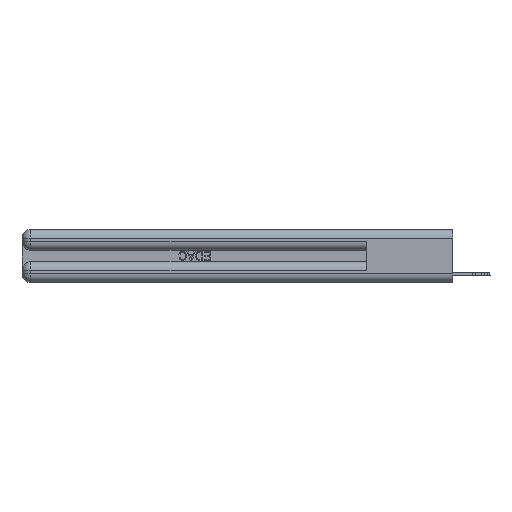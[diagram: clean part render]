
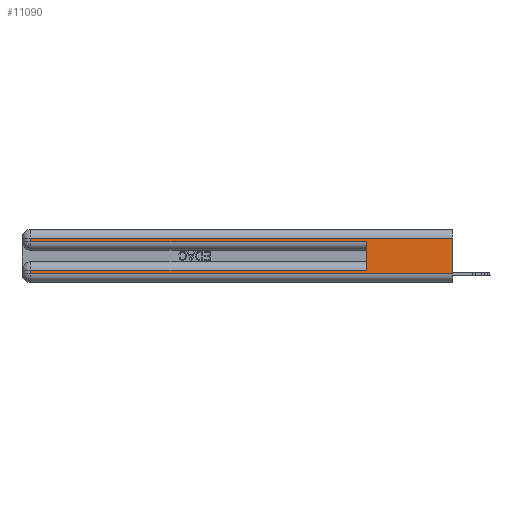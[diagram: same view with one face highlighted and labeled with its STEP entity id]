
A CAD part, left-side view. The second image highlights one B-rep face of the part: STEP entity #11090.
In plain terms, the highlighted planar face has unit normal (-1, 0, 0).
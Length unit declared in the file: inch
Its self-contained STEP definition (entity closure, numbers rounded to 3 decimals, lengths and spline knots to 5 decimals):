
#263 = CARTESIAN_POINT ( 'NONE',  ( 0., 0., 0.285 ) ) ;
#1308 = ORIENTED_EDGE ( 'NONE', *, *, #21689, .T. ) ;
#2280 = DIRECTION ( 'NONE',  ( 0., 1., 0. ) ) ;
#2573 = ORIENTED_EDGE ( 'NONE', *, *, #19271, .F. ) ;
#2733 = VECTOR ( 'NONE', #10560, 39.37008 ) ;
#3827 = CARTESIAN_POINT ( 'NONE',  ( 0., 2.94, 0.37 ) ) ;
#4783 = ORIENTED_EDGE ( 'NONE', *, *, #11124, .T. ) ;
#4931 = DIRECTION ( 'NONE',  ( 0., 0., -1. ) ) ;
#5399 = CARTESIAN_POINT ( 'NONE',  ( 0., 0., 0.06 ) ) ;
#5500 = VERTEX_POINT ( 'NONE', #27693 ) ;
#5963 = VECTOR ( 'NONE', #8279, 39.37008 ) ;
#7023 = CARTESIAN_POINT ( 'NONE',  ( 0., 0., 0.37 ) ) ;
#7099 = CARTESIAN_POINT ( 'NONE',  ( 0., 2.94, 0.37 ) ) ;
#8279 = DIRECTION ( 'NONE',  ( 0., 0., 1. ) ) ;
#8488 = VECTOR ( 'NONE', #12226, 39.37008 ) ;
#8755 = LINE ( 'NONE', #18513, #5963 ) ;
#8760 = VECTOR ( 'NONE', #2280, 39.37008 ) ;
#10560 = DIRECTION ( 'NONE',  ( 0., 1., 0. ) ) ;
#11020 = VERTEX_POINT ( 'NONE', #23036 ) ;
#11090 = ADVANCED_FACE ( 'NONE', ( #18244 ), #15538, .F. ) ;
#11124 = EDGE_CURVE ( 'NONE', #5500, #11020, #12974, .T. ) ;
#12226 = DIRECTION ( 'NONE',  ( 0., 0., -1. ) ) ;
#12974 = LINE ( 'NONE', #22556, #2733 ) ;
#13335 = ORIENTED_EDGE ( 'NONE', *, *, #22567, .T. ) ;
#13563 = EDGE_CURVE ( 'NONE', #30254, #25955, #14953, .T. ) ;
#14432 = CARTESIAN_POINT ( 'NONE',  ( 0., 2.94, 0.285 ) ) ;
#14953 = LINE ( 'NONE', #7099, #8488 ) ;
#15154 = VERTEX_POINT ( 'NONE', #22585 ) ;
#15222 = EDGE_CURVE ( 'NONE', #25955, #22639, #30396, .T. ) ;
#15402 = ORIENTED_EDGE ( 'NONE', *, *, #15222, .T. ) ;
#15538 = PLANE ( 'NONE',  #28278 ) ;
#16202 = EDGE_CURVE ( 'NONE', #15154, #21276, #8755, .T. ) ;
#17010 = EDGE_CURVE ( 'NONE', #11020, #22063, #25745, .T. ) ;
#17110 = DIRECTION ( 'NONE',  ( 0., -1., 0. ) ) ;
#18120 = EDGE_LOOP ( 'NONE', ( #2573, #4783, #28640, #13335, #25942, #1308, #27802, #15402 ) ) ;
#18244 = FACE_OUTER_BOUND ( 'NONE', #18120, .T. ) ;
#18513 = CARTESIAN_POINT ( 'NONE',  ( 0., 0.6, 0.145 ) ) ;
#18586 = CARTESIAN_POINT ( 'NONE',  ( 0., 0., 0.06 ) ) ;
#19181 = LINE ( 'NONE', #7023, #30069 ) ;
#19271 = EDGE_CURVE ( 'NONE', #5500, #22639, #19181, .T. ) ;
#19563 = LINE ( 'NONE', #24206, #8760 ) ;
#19778 = VECTOR ( 'NONE', #28012, 39.37008 ) ;
#21276 = VERTEX_POINT ( 'NONE', #24384 ) ;
#21689 = EDGE_CURVE ( 'NONE', #15154, #30254, #19563, .T. ) ;
#21897 = CARTESIAN_POINT ( 'NONE',  ( 0., 2.94, 0.085 ) ) ;
#22063 = VERTEX_POINT ( 'NONE', #14432 ) ;
#22556 = CARTESIAN_POINT ( 'NONE',  ( 0., 0., 0.31 ) ) ;
#22567 = EDGE_CURVE ( 'NONE', #22063, #21276, #24614, .T. ) ;
#22585 = CARTESIAN_POINT ( 'NONE',  ( 0., 0.6, 0.085 ) ) ;
#22639 = VERTEX_POINT ( 'NONE', #5399 ) ;
#23036 = CARTESIAN_POINT ( 'NONE',  ( 0., 2.94, 0.31 ) ) ;
#23343 = VECTOR ( 'NONE', #28295, 39.37008 ) ;
#24206 = CARTESIAN_POINT ( 'NONE',  ( 0., 0., 0.085 ) ) ;
#24384 = CARTESIAN_POINT ( 'NONE',  ( 0., 0.6, 0.285 ) ) ;
#24614 = LINE ( 'NONE', #263, #24903 ) ;
#24903 = VECTOR ( 'NONE', #17110, 39.37008 ) ;
#24953 = DIRECTION ( 'NONE',  ( 0., 0., -1. ) ) ;
#25745 = LINE ( 'NONE', #3827, #23343 ) ;
#25942 = ORIENTED_EDGE ( 'NONE', *, *, #16202, .F. ) ;
#25955 = VERTEX_POINT ( 'NONE', #29059 ) ;
#27693 = CARTESIAN_POINT ( 'NONE',  ( 0., 0., 0.31 ) ) ;
#27802 = ORIENTED_EDGE ( 'NONE', *, *, #13563, .T. ) ;
#27982 = DIRECTION ( 'NONE',  ( 1., 0., 0. ) ) ;
#28012 = DIRECTION ( 'NONE',  ( 0., -1., 0. ) ) ;
#28278 = AXIS2_PLACEMENT_3D ( 'NONE', #30043, #27982, #24953 ) ;
#28295 = DIRECTION ( 'NONE',  ( 0., 0., -1. ) ) ;
#28640 = ORIENTED_EDGE ( 'NONE', *, *, #17010, .T. ) ;
#29059 = CARTESIAN_POINT ( 'NONE',  ( 0., 2.94, 0.06 ) ) ;
#30043 = CARTESIAN_POINT ( 'NONE',  ( 0., 0., 0.37 ) ) ;
#30069 = VECTOR ( 'NONE', #4931, 39.37008 ) ;
#30254 = VERTEX_POINT ( 'NONE', #21897 ) ;
#30396 = LINE ( 'NONE', #18586, #19778 ) ;
